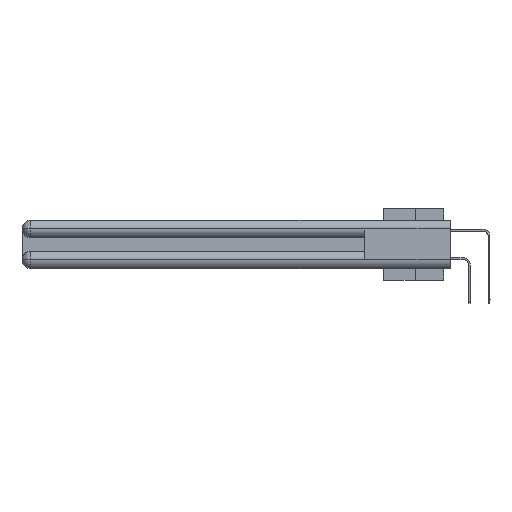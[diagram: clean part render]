
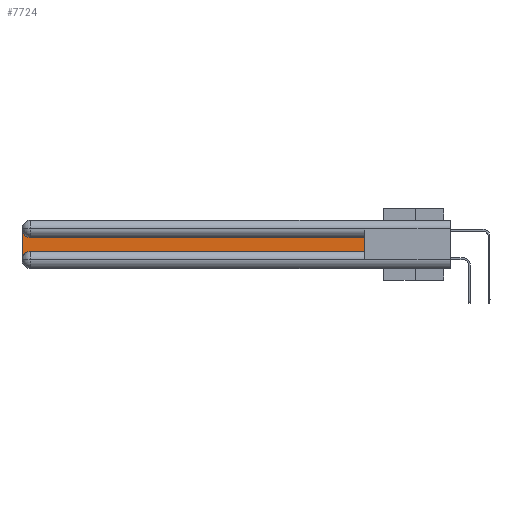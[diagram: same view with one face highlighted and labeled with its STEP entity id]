
A CAD part, left-side view. The second image highlights one B-rep face of the part: STEP entity #7724.
In plain terms, the highlighted planar face has unit normal (-1, 0, 0).
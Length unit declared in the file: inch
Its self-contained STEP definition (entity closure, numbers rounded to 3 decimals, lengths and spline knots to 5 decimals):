
#718 = CARTESIAN_POINT ( 'NONE',  ( 0.075, 3., -0.1225 ) ) ;
#4040 = CARTESIAN_POINT ( 'NONE',  ( 0.075, 3., -0.2775 ) ) ;
#4515 = LINE ( 'NONE', #15442, #11886 ) ;
#4724 = ORIENTED_EDGE ( 'NONE', *, *, #23972, .T. ) ;
#6403 = VERTEX_POINT ( 'NONE', #16108 ) ;
#7481 = DIRECTION ( 'NONE',  ( 1., 0., 0. ) ) ;
#7651 = CARTESIAN_POINT ( 'NONE',  ( 0.075, 2.94, -0.0625 ) ) ;
#7724 = ADVANCED_FACE ( 'NONE', ( #14325 ), #25232, .F. ) ;
#9202 = DIRECTION ( 'NONE',  ( 1., 0., 0. ) ) ;
#10250 = CIRCLE ( 'NONE', #11974, 0.06 ) ;
#10290 = DIRECTION ( 'NONE',  ( 0., 0., 1. ) ) ;
#10558 = CARTESIAN_POINT ( 'NONE',  ( 0.075, 0.6, -0.2175 ) ) ;
#11268 = LINE ( 'NONE', #10558, #26281 ) ;
#11886 = VECTOR ( 'NONE', #31681, 39.37008 ) ;
#11974 = AXIS2_PLACEMENT_3D ( 'NONE', #33332, #9202, #28165 ) ;
#13213 = EDGE_CURVE ( 'NONE', #23739, #25465, #4515, .T. ) ;
#14325 = FACE_OUTER_BOUND ( 'NONE', #31549, .T. ) ;
#14609 = CARTESIAN_POINT ( 'NONE',  ( 0.075, 3., -0.0625 ) ) ;
#14859 = DIRECTION ( 'NONE',  ( 0., 1., 0. ) ) ;
#15442 = CARTESIAN_POINT ( 'NONE',  ( 0.075, 3., -0.2175 ) ) ;
#16108 = CARTESIAN_POINT ( 'NONE',  ( 0.075, 0.6, -0.1225 ) ) ;
#18656 = EDGE_CURVE ( 'NONE', #6403, #27028, #25128, .T. ) ;
#18952 = DIRECTION ( 'NONE',  ( 0., 0., -1. ) ) ;
#19071 = ORIENTED_EDGE ( 'NONE', *, *, #18656, .T. ) ;
#19197 = CARTESIAN_POINT ( 'NONE',  ( 0.075, 0.6, -0.1225 ) ) ;
#20979 = ORIENTED_EDGE ( 'NONE', *, *, #31016, .T. ) ;
#21373 = AXIS2_PLACEMENT_3D ( 'NONE', #718, #33419, #18952 ) ;
#22181 = DIRECTION ( 'NONE',  ( 0., -1., 0. ) ) ;
#22921 = VERTEX_POINT ( 'NONE', #32405 ) ;
#23153 = VERTEX_POINT ( 'NONE', #24573 ) ;
#23739 = VERTEX_POINT ( 'NONE', #14609 ) ;
#23917 = LINE ( 'NONE', #34774, #27319 ) ;
#23972 = EDGE_CURVE ( 'NONE', #22921, #6403, #23917, .T. ) ;
#24127 = ORIENTED_EDGE ( 'NONE', *, *, #31437, .T. ) ;
#24573 = CARTESIAN_POINT ( 'NONE',  ( 0.075, 2.94, -0.2175 ) ) ;
#25068 = ORIENTED_EDGE ( 'NONE', *, *, #13213, .T. ) ;
#25128 = LINE ( 'NONE', #19197, #34557 ) ;
#25232 = PLANE ( 'NONE',  #21373 ) ;
#25465 = VERTEX_POINT ( 'NONE', #4040 ) ;
#26281 = VECTOR ( 'NONE', #22181, 39.37008 ) ;
#27028 = VERTEX_POINT ( 'NONE', #34779 ) ;
#27319 = VECTOR ( 'NONE', #10290, 39.37008 ) ;
#28165 = DIRECTION ( 'NONE',  ( 0., 0., -1. ) ) ;
#29123 = DIRECTION ( 'NONE',  ( 0., 0., -1. ) ) ;
#30274 = CIRCLE ( 'NONE', #31342, 0.06 ) ;
#30747 = EDGE_CURVE ( 'NONE', #23153, #22921, #11268, .T. ) ;
#30943 = ORIENTED_EDGE ( 'NONE', *, *, #30747, .T. ) ;
#31016 = EDGE_CURVE ( 'NONE', #27028, #23739, #30274, .T. ) ;
#31342 = AXIS2_PLACEMENT_3D ( 'NONE', #7651, #7481, #29123 ) ;
#31437 = EDGE_CURVE ( 'NONE', #25465, #23153, #10250, .T. ) ;
#31549 = EDGE_LOOP ( 'NONE', ( #19071, #20979, #25068, #24127, #30943, #4724 ) ) ;
#31681 = DIRECTION ( 'NONE',  ( 0., 0., -1. ) ) ;
#32405 = CARTESIAN_POINT ( 'NONE',  ( 0.075, 0.6, -0.2175 ) ) ;
#33332 = CARTESIAN_POINT ( 'NONE',  ( 0.075, 2.94, -0.2775 ) ) ;
#33419 = DIRECTION ( 'NONE',  ( 1., 0., 0. ) ) ;
#34557 = VECTOR ( 'NONE', #14859, 39.37008 ) ;
#34774 = CARTESIAN_POINT ( 'NONE',  ( 0.075, 0.6, -0.2175 ) ) ;
#34779 = CARTESIAN_POINT ( 'NONE',  ( 0.075, 2.94, -0.1225 ) ) ;
